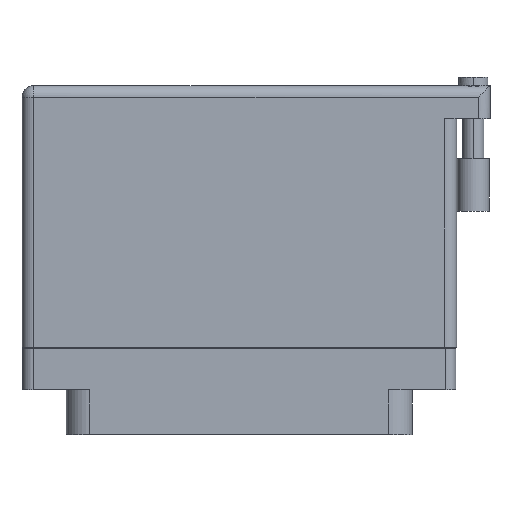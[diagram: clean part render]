
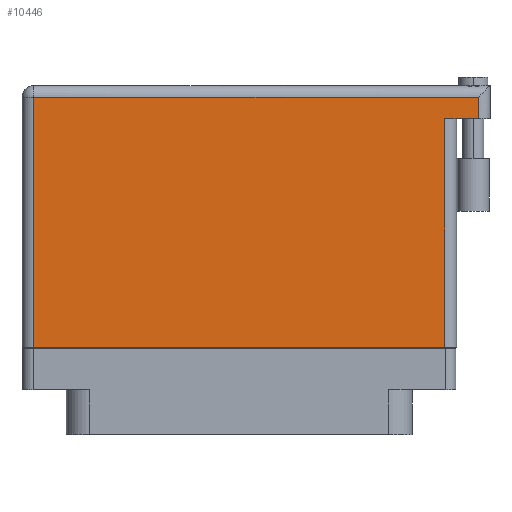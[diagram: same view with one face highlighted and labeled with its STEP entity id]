
A CAD part, front view. The second image highlights one B-rep face of the part: STEP entity #10446.
In plain terms, the highlighted face is planar.
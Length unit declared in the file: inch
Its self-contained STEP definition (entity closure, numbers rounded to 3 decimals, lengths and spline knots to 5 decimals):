
#3029 = DIRECTION ( 'NONE',  ( 0., 1., 0. ) ) ;
#3724 = CARTESIAN_POINT ( 'NONE',  ( -1.3, 1.466, 0.4495 ) ) ;
#4216 = DIRECTION ( 'NONE',  ( 0., 0., -1. ) ) ;
#5829 = LINE ( 'NONE', #46255, #47260 ) ;
#6237 = CARTESIAN_POINT ( 'NONE',  ( -1.3, 1.396, 0.4495 ) ) ;
#6407 = CARTESIAN_POINT ( 'NONE',  ( -1.3, -0.1, 0.4495 ) ) ;
#6813 = VERTEX_POINT ( 'NONE', #21366 ) ;
#6875 = DIRECTION ( 'NONE',  ( 1., 0., 0. ) ) ;
#7668 = ORIENTED_EDGE ( 'NONE', *, *, #20309, .T. ) ;
#8353 = FACE_OUTER_BOUND ( 'NONE', #29532, .T. ) ;
#10446 = ADVANCED_FACE ( 'NONE', ( #8353 ), #18210, .F. ) ;
#12772 = DIRECTION ( 'NONE',  ( 0., -1., 0. ) ) ;
#13849 = LINE ( 'NONE', #39389, #16713 ) ;
#15335 = EDGE_CURVE ( 'NONE', #43083, #22569, #35918, .T. ) ;
#16281 = ORIENTED_EDGE ( 'NONE', *, *, #18741, .T. ) ;
#16713 = VECTOR ( 'NONE', #3029, 39.37008 ) ;
#17620 = CARTESIAN_POINT ( 'NONE',  ( 1.43, 1.269, 0.4495 ) ) ;
#17807 = EDGE_CURVE ( 'NONE', #22569, #18052, #5829, .T. ) ;
#18052 = VERTEX_POINT ( 'NONE', #36450 ) ;
#18210 = PLANE ( 'NONE',  #34977 ) ;
#18388 = LINE ( 'NONE', #38627, #25874 ) ;
#18741 = EDGE_CURVE ( 'NONE', #18052, #6813, #26121, .T. ) ;
#20110 = VECTOR ( 'NONE', #27687, 39.37008 ) ;
#20309 = EDGE_CURVE ( 'NONE', #6813, #22411, #13849, .T. ) ;
#21366 = CARTESIAN_POINT ( 'NONE',  ( 1.23, -0.1, 0.4495 ) ) ;
#22411 = VERTEX_POINT ( 'NONE', #33344 ) ;
#22569 = VERTEX_POINT ( 'NONE', #32216 ) ;
#23125 = ORIENTED_EDGE ( 'NONE', *, *, #15335, .T. ) ;
#23971 = CARTESIAN_POINT ( 'NONE',  ( 1.5, 1.269, 0.4495 ) ) ;
#25874 = VECTOR ( 'NONE', #46653, 39.37008 ) ;
#26121 = LINE ( 'NONE', #6407, #38224 ) ;
#26123 = VECTOR ( 'NONE', #32340, 39.37008 ) ;
#27687 = DIRECTION ( 'NONE',  ( -1., 0., 0. ) ) ;
#29532 = EDGE_LOOP ( 'NONE', ( #16281, #7668, #37414, #39590, #23125, #42090 ) ) ;
#29910 = LINE ( 'NONE', #23971, #20110 ) ;
#32216 = CARTESIAN_POINT ( 'NONE',  ( -1.23, 1.396, 0.4495 ) ) ;
#32340 = DIRECTION ( 'NONE',  ( -1., 0., 0. ) ) ;
#33166 = DIRECTION ( 'NONE',  ( -1., 0., 0. ) ) ;
#33344 = CARTESIAN_POINT ( 'NONE',  ( 1.23, 1.269, 0.4495 ) ) ;
#34977 = AXIS2_PLACEMENT_3D ( 'NONE', #3724, #4216, #33166 ) ;
#35918 = LINE ( 'NONE', #6237, #26123 ) ;
#36450 = CARTESIAN_POINT ( 'NONE',  ( -1.23, -0.1, 0.4495 ) ) ;
#37414 = ORIENTED_EDGE ( 'NONE', *, *, #38832, .F. ) ;
#38224 = VECTOR ( 'NONE', #6875, 39.37008 ) ;
#38627 = CARTESIAN_POINT ( 'NONE',  ( 1.43, 1.466, 0.4495 ) ) ;
#38832 = EDGE_CURVE ( 'NONE', #39300, #22411, #29910, .T. ) ;
#39300 = VERTEX_POINT ( 'NONE', #17620 ) ;
#39389 = CARTESIAN_POINT ( 'NONE',  ( 1.23, 1.269, 0.4495 ) ) ;
#39590 = ORIENTED_EDGE ( 'NONE', *, *, #47287, .T. ) ;
#42090 = ORIENTED_EDGE ( 'NONE', *, *, #17807, .T. ) ;
#43083 = VERTEX_POINT ( 'NONE', #44000 ) ;
#44000 = CARTESIAN_POINT ( 'NONE',  ( 1.43, 1.396, 0.4495 ) ) ;
#46255 = CARTESIAN_POINT ( 'NONE',  ( -1.23, -0.1, 0.4495 ) ) ;
#46653 = DIRECTION ( 'NONE',  ( 0., 1., 0. ) ) ;
#47260 = VECTOR ( 'NONE', #12772, 39.37008 ) ;
#47287 = EDGE_CURVE ( 'NONE', #39300, #43083, #18388, .T. ) ;
